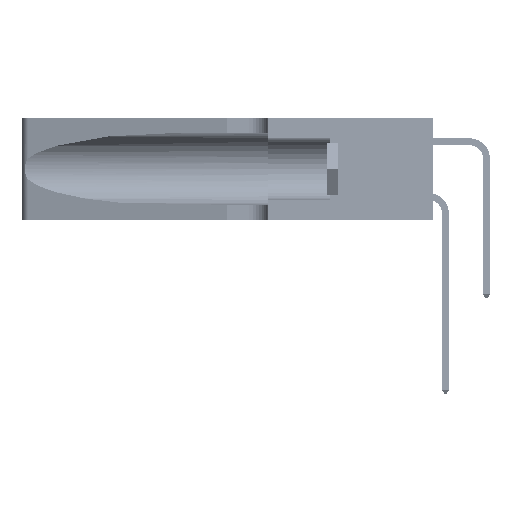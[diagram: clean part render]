
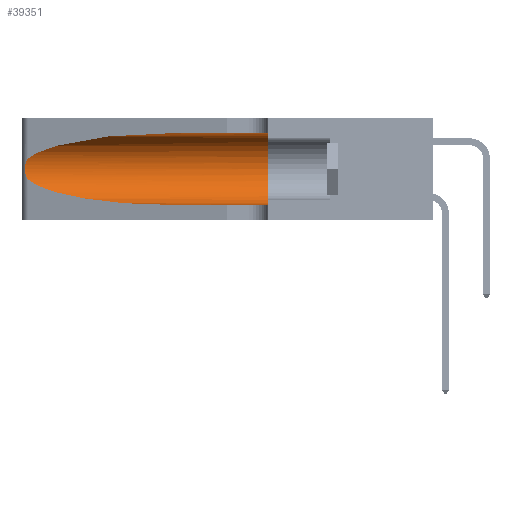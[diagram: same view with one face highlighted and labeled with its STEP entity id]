
A CAD part, left-side view. The second image highlights one B-rep face of the part: STEP entity #39351.
In plain terms, the highlighted cylindrical face has radius 3.308 mm (diameter 6.617 mm), a partial arc.
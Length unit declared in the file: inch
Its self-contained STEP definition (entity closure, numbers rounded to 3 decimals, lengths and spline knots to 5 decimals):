
#28 = CARTESIAN_POINT ( 'NONE',  ( 0.1305, 1.61858, 0.185 ) ) ;
#3453 = CARTESIAN_POINT ( 'NONE',  ( 0.1305, 0.72297, 0.31525 ) ) ;
#3583 = CARTESIAN_POINT ( 'NONE',  ( 0.25787, 1.23484, 0.2124 ) ) ;
#4305 = ORIENTED_EDGE ( 'NONE', *, *, #22604, .T. ) ;
#5421 = CARTESIAN_POINT ( 'NONE',  ( 0.25487, 1.22718, 0.14631 ) ) ;
#7338 = DIRECTION ( 'NONE',  ( 0., 0., 1. ) ) ;
#7409 = CARTESIAN_POINT ( 'NONE',  ( 0.26075, 1.23896, 0.178 ) ) ;
#7560 = CARTESIAN_POINT ( 'NONE',  ( 0.25639, 1.23184, 0.21858 ) ) ;
#7826 = LINE ( 'NONE', #44745, #38664 ) ;
#7910 = CARTESIAN_POINT ( 'NONE',  ( 0.25487, 1.22718, 0.22369 ) ) ;
#8095 = ORIENTED_EDGE ( 'NONE', *, *, #21888, .T. ) ;
#8895 = CARTESIAN_POINT ( 'NONE',  ( 0.25487, 1.22718, 0.22369 ) ) ;
#9203 = CARTESIAN_POINT ( 'NONE',  ( 0.1305, 0.35, 0.31525 ) ) ;
#11085 = CARTESIAN_POINT ( 'NONE',  ( 0.1305, 0.72297, 0.05475 ) ) ;
#11650 = CIRCLE ( 'NONE', #23300, 0.13025 ) ;
#11961 = CARTESIAN_POINT ( 'NONE',  ( 0.25487, 1.22718, 0.14631 ) ) ;
#12160 = DIRECTION ( 'NONE',  ( 0., -1., 0. ) ) ;
#12788 = VERTEX_POINT ( 'NONE', #45264 ) ;
#14634 = CARTESIAN_POINT ( 'NONE',  ( 0.26075, 1.23896, 0.19203 ) ) ;
#14731 = EDGE_CURVE ( 'NONE', #28501, #21820, #16307, .T. ) ;
#14949 = CARTESIAN_POINT ( 'NONE',  ( 0.25555, 1.22993, 0.14849 ) ) ;
#16307 =( BOUNDED_CURVE ( )  B_SPLINE_CURVE ( 3, ( #11961, #44711, #19329, #44863 ),
 .UNSPECIFIED., .F., .F. ) 
 B_SPLINE_CURVE_WITH_KNOTS ( ( 4, 4 ),
 ( 3.44316, 4.71239 ),
 .UNSPECIFIED. ) 
 CURVE ( )  GEOMETRIC_REPRESENTATION_ITEM ( )  RATIONAL_B_SPLINE_CURVE ( ( 1., 0.87, 0.87, 1. ) ) 
 REPRESENTATION_ITEM ( '' )  );
#16792 = CYLINDRICAL_SURFACE ( 'NONE', #29006, 0.13025 ) ;
#16836 = ORIENTED_EDGE ( 'NONE', *, *, #40938, .F. ) ;
#16857 = VERTEX_POINT ( 'NONE', #9203 ) ;
#16980 = CARTESIAN_POINT ( 'NONE',  ( 0.1305, 1.61858, 0.31525 ) ) ;
#17408 = VERTEX_POINT ( 'NONE', #44942 ) ;
#18004 = CARTESIAN_POINT ( 'NONE',  ( 0.25856, 1.23593, 0.16098 ) ) ;
#19329 = CARTESIAN_POINT ( 'NONE',  ( 0.18966, 0.96281, 0.05475 ) ) ;
#21820 = VERTEX_POINT ( 'NONE', #11085 ) ;
#21888 = EDGE_CURVE ( 'NONE', #43857, #28501, #31168, .T. ) ;
#22604 = EDGE_CURVE ( 'NONE', #21820, #17408, #7826, .T. ) ;
#23300 = AXIS2_PLACEMENT_3D ( 'NONE', #29326, #33342, #7338 ) ;
#25353 = CARTESIAN_POINT ( 'NONE',  ( 0.25789, 1.23486, 0.15765 ) ) ;
#26152 = CARTESIAN_POINT ( 'NONE',  ( 0.2373, 1.15595, 0.28018 ) ) ;
#26488 = FACE_OUTER_BOUND ( 'NONE', #28121, .T. ) ;
#27147 = ORIENTED_EDGE ( 'NONE', *, *, #32762, .T. ) ;
#28121 = EDGE_LOOP ( 'NONE', ( #27147, #8095, #28710, #4305, #16836, #43804 ) ) ;
#28501 = VERTEX_POINT ( 'NONE', #5421 ) ;
#28710 = ORIENTED_EDGE ( 'NONE', *, *, #14731, .T. ) ;
#29006 = AXIS2_PLACEMENT_3D ( 'NONE', #28, #36690, #32775 ) ;
#29281 = CARTESIAN_POINT ( 'NONE',  ( 0.26017, 1.23833, 0.17102 ) ) ;
#29326 = CARTESIAN_POINT ( 'NONE',  ( 0.1305, 0.35, 0.185 ) ) ;
#29451 = CARTESIAN_POINT ( 'NONE',  ( 0.25555, 1.22994, 0.2215 ) ) ;
#29819 = VECTOR ( 'NONE', #39672, 39.37008 ) ;
#31168 = B_SPLINE_CURVE_WITH_KNOTS ( 'NONE', 3,
 ( #47050, #29451, #7560, #3583, #36226, #36388, #14634, #7409, #29281, #18004, #25353, #33099, #14949, #40072 ),
 .UNSPECIFIED., .F., .F.,
 ( 4, 2, 2, 2, 2, 2, 4 ),
 ( 0., 0.00027, 0.00053, 0.00107, 0.0016, 0.00187, 0.00214 ),
 .UNSPECIFIED. ) ;
#32762 = EDGE_CURVE ( 'NONE', #12788, #43857, #46538, .T. ) ;
#32775 = DIRECTION ( 'NONE',  ( 0., 0., -1. ) ) ;
#33099 = CARTESIAN_POINT ( 'NONE',  ( 0.25639, 1.23186, 0.15144 ) ) ;
#33127 = CARTESIAN_POINT ( 'NONE',  ( 0.18966, 0.96281, 0.31525 ) ) ;
#33342 = DIRECTION ( 'NONE',  ( 0., 1., 0. ) ) ;
#36226 = CARTESIAN_POINT ( 'NONE',  ( 0.25854, 1.2359, 0.20912 ) ) ;
#36388 = CARTESIAN_POINT ( 'NONE',  ( 0.26018, 1.23835, 0.19895 ) ) ;
#36690 = DIRECTION ( 'NONE',  ( 0., -1., 0. ) ) ;
#38664 = VECTOR ( 'NONE', #12160, 39.37008 ) ;
#39351 = ADVANCED_FACE ( 'NONE', ( #26488 ), #16792, .F. ) ;
#39672 = DIRECTION ( 'NONE',  ( 0., -1., 0. ) ) ;
#40072 = CARTESIAN_POINT ( 'NONE',  ( 0.25487, 1.22718, 0.14631 ) ) ;
#40938 = EDGE_CURVE ( 'NONE', #16857, #17408, #11650, .T. ) ;
#41600 = LINE ( 'NONE', #16980, #29819 ) ;
#43804 = ORIENTED_EDGE ( 'NONE', *, *, #45334, .F. ) ;
#43857 = VERTEX_POINT ( 'NONE', #8895 ) ;
#44711 = CARTESIAN_POINT ( 'NONE',  ( 0.2373, 1.15595, 0.08982 ) ) ;
#44745 = CARTESIAN_POINT ( 'NONE',  ( 0.1305, 1.61858, 0.05475 ) ) ;
#44863 = CARTESIAN_POINT ( 'NONE',  ( 0.1305, 0.72297, 0.05475 ) ) ;
#44942 = CARTESIAN_POINT ( 'NONE',  ( 0.1305, 0.35, 0.05475 ) ) ;
#45264 = CARTESIAN_POINT ( 'NONE',  ( 0.1305, 0.72297, 0.31525 ) ) ;
#45334 = EDGE_CURVE ( 'NONE', #12788, #16857, #41600, .T. ) ;
#46538 =( BOUNDED_CURVE ( )  B_SPLINE_CURVE ( 3, ( #3453, #33127, #26152, #7910 ),
 .UNSPECIFIED., .F., .T. ) 
 B_SPLINE_CURVE_WITH_KNOTS ( ( 4, 4 ),
 ( 1.5708, 2.84003 ),
 .UNSPECIFIED. ) 
 CURVE ( )  GEOMETRIC_REPRESENTATION_ITEM ( )  RATIONAL_B_SPLINE_CURVE ( ( 1., 0.87, 0.87, 1. ) ) 
 REPRESENTATION_ITEM ( '' )  );
#47050 = CARTESIAN_POINT ( 'NONE',  ( 0.25487, 1.22718, 0.22369 ) ) ;
